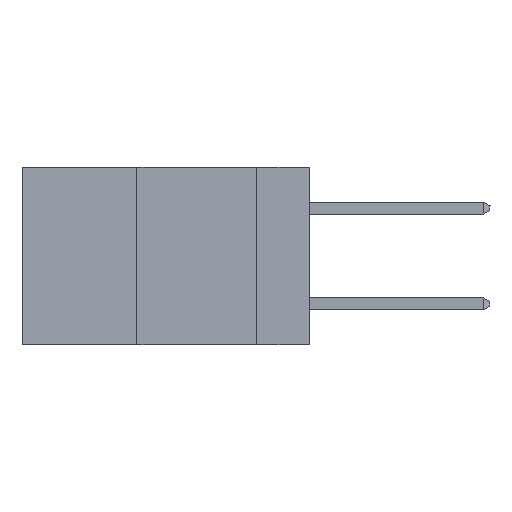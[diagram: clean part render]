
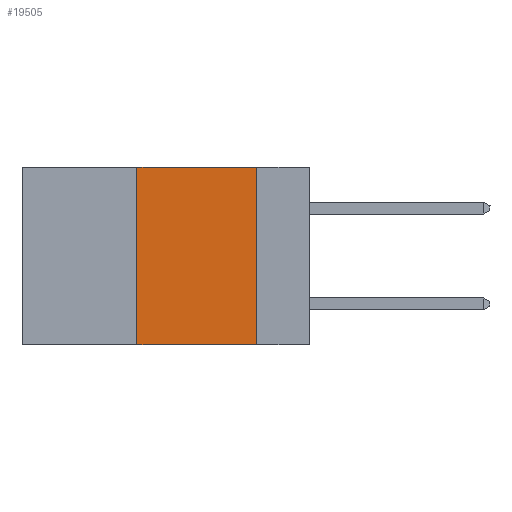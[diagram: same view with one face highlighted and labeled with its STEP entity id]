
A CAD part, left-side view. The second image highlights one B-rep face of the part: STEP entity #19505.
In plain terms, the highlighted planar face has unit normal (-1, 0, 0).
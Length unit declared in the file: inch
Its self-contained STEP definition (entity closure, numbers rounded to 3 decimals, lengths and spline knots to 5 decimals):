
#267 = DIRECTION ( 'NONE',  ( 0., -1., 0. ) ) ;
#784 = EDGE_CURVE ( 'NONE', #30363, #23809, #32026, .T. ) ;
#1147 = CARTESIAN_POINT ( 'NONE',  ( 0., 0.11, 0. ) ) ;
#1994 = DIRECTION ( 'NONE',  ( 0., -1., 0. ) ) ;
#2228 = CARTESIAN_POINT ( 'NONE',  ( 0., 0.6, 0. ) ) ;
#5434 = ORIENTED_EDGE ( 'NONE', *, *, #36891, .F. ) ;
#5472 = EDGE_CURVE ( 'NONE', #18081, #23809, #30690, .T. ) ;
#6782 = ORIENTED_EDGE ( 'NONE', *, *, #784, .T. ) ;
#9024 = CARTESIAN_POINT ( 'NONE',  ( 0., 0.36, 0. ) ) ;
#11284 = PLANE ( 'NONE',  #16853 ) ;
#12253 = CARTESIAN_POINT ( 'NONE',  ( 0., 0.11, 0. ) ) ;
#13593 = CARTESIAN_POINT ( 'NONE',  ( 0., 0.36, -0.37 ) ) ;
#14284 = DIRECTION ( 'NONE',  ( 1., 0., 0. ) ) ;
#14663 = LINE ( 'NONE', #35747, #29419 ) ;
#15006 = CARTESIAN_POINT ( 'NONE',  ( 0., 0.6, -0.37 ) ) ;
#16381 = VECTOR ( 'NONE', #1994, 39.37008 ) ;
#16389 = DIRECTION ( 'NONE',  ( 0., 0., 1. ) ) ;
#16576 = VECTOR ( 'NONE', #16389, 39.37008 ) ;
#16853 = AXIS2_PLACEMENT_3D ( 'NONE', #2228, #14284, #34843 ) ;
#18081 = VERTEX_POINT ( 'NONE', #1147 ) ;
#19505 = ADVANCED_FACE ( 'NONE', ( #36094 ), #11284, .F. ) ;
#23160 = ORIENTED_EDGE ( 'NONE', *, *, #5472, .F. ) ;
#23809 = VERTEX_POINT ( 'NONE', #26715 ) ;
#24054 = EDGE_LOOP ( 'NONE', ( #23160, #5434, #31334, #6782 ) ) ;
#24452 = LINE ( 'NONE', #31050, #16576 ) ;
#25479 = EDGE_CURVE ( 'NONE', #30363, #32656, #24452, .T. ) ;
#26715 = CARTESIAN_POINT ( 'NONE',  ( 0., 0.11, -0.37 ) ) ;
#29419 = VECTOR ( 'NONE', #267, 39.37008 ) ;
#29935 = DIRECTION ( 'NONE',  ( 0., 0., -1. ) ) ;
#30363 = VERTEX_POINT ( 'NONE', #13593 ) ;
#30690 = LINE ( 'NONE', #12253, #37505 ) ;
#31050 = CARTESIAN_POINT ( 'NONE',  ( 0., 0.36, 0. ) ) ;
#31334 = ORIENTED_EDGE ( 'NONE', *, *, #25479, .F. ) ;
#32026 = LINE ( 'NONE', #15006, #16381 ) ;
#32656 = VERTEX_POINT ( 'NONE', #9024 ) ;
#34843 = DIRECTION ( 'NONE',  ( 0., 0., -1. ) ) ;
#35747 = CARTESIAN_POINT ( 'NONE',  ( 0., 0.6, 0. ) ) ;
#36094 = FACE_OUTER_BOUND ( 'NONE', #24054, .T. ) ;
#36891 = EDGE_CURVE ( 'NONE', #32656, #18081, #14663, .T. ) ;
#37505 = VECTOR ( 'NONE', #29935, 39.37008 ) ;
